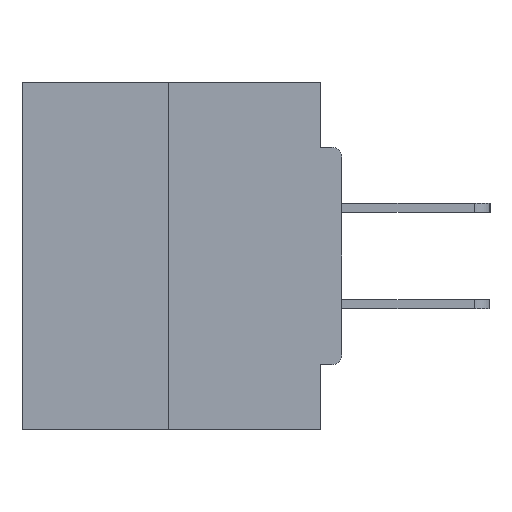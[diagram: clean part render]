
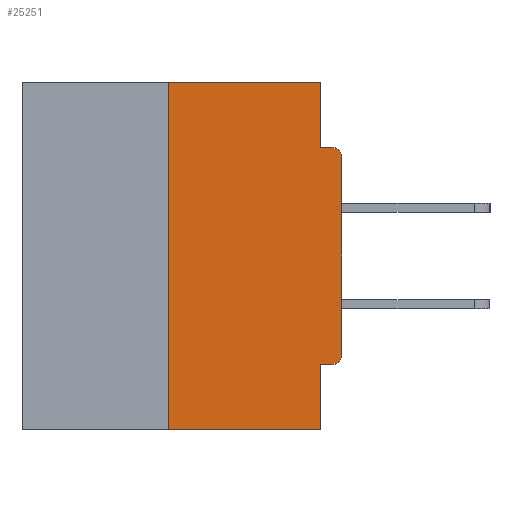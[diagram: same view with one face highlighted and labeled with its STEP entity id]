
A CAD part, left-side view. The second image highlights one B-rep face of the part: STEP entity #25251.
In plain terms, the highlighted planar face has unit normal (-1, 0, 0).
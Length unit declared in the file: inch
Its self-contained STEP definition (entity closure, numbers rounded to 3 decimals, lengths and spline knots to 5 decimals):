
#108 = ORIENTED_EDGE ( 'NONE', *, *, #28873, .F. ) ;
#374 = VERTEX_POINT ( 'NONE', #25439 ) ;
#967 = VECTOR ( 'NONE', #21039, 39.37008 ) ;
#1845 = VERTEX_POINT ( 'NONE', #27492 ) ;
#2321 = LINE ( 'NONE', #20231, #15808 ) ;
#3077 = AXIS2_PLACEMENT_3D ( 'NONE', #6967, #7085, #28451 ) ;
#3712 = CARTESIAN_POINT ( 'NONE',  ( 0., 0.015, -0.4065 ) ) ;
#3963 = VERTEX_POINT ( 'NONE', #11438 ) ;
#4466 = CARTESIAN_POINT ( 'NONE',  ( 0., 0.25, 0. ) ) ;
#4668 = VECTOR ( 'NONE', #16037, 39.37008 ) ;
#4736 = LINE ( 'NONE', #13204, #967 ) ;
#4924 = EDGE_CURVE ( 'NONE', #24156, #24502, #10469, .T. ) ;
#5643 = DIRECTION ( 'NONE',  ( 0., 0., -1. ) ) ;
#5819 = DIRECTION ( 'NONE',  ( -1., 0., 0. ) ) ;
#5841 = VECTOR ( 'NONE', #5643, 39.37008 ) ;
#5943 = DIRECTION ( 'NONE',  ( 0., 0., 1. ) ) ;
#6967 = CARTESIAN_POINT ( 'NONE',  ( 0., 0.015, -0.1085 ) ) ;
#7085 = DIRECTION ( 'NONE',  ( -1., 0., 0. ) ) ;
#8122 = VERTEX_POINT ( 'NONE', #13947 ) ;
#8282 = ORIENTED_EDGE ( 'NONE', *, *, #14722, .T. ) ;
#8431 = LINE ( 'NONE', #8628, #26182 ) ;
#8519 = EDGE_CURVE ( 'NONE', #18077, #1845, #4736, .T. ) ;
#8626 = CARTESIAN_POINT ( 'NONE',  ( 0., 0.031, -0.5 ) ) ;
#8628 = CARTESIAN_POINT ( 'NONE',  ( 0., 0., -0.0935 ) ) ;
#9021 = ORIENTED_EDGE ( 'NONE', *, *, #8519, .F. ) ;
#9409 = ORIENTED_EDGE ( 'NONE', *, *, #18196, .T. ) ;
#9428 = EDGE_CURVE ( 'NONE', #374, #25283, #22855, .T. ) ;
#10469 = LINE ( 'NONE', #32839, #5841 ) ;
#10482 = ORIENTED_EDGE ( 'NONE', *, *, #20286, .F. ) ;
#10973 = CARTESIAN_POINT ( 'NONE',  ( 0., 0.25, 0. ) ) ;
#11276 = CARTESIAN_POINT ( 'NONE',  ( 0., 0., -0.3915 ) ) ;
#11438 = CARTESIAN_POINT ( 'NONE',  ( 0., 0.015, -0.0935 ) ) ;
#12841 = DIRECTION ( 'NONE',  ( 0., 0., -1. ) ) ;
#13204 = CARTESIAN_POINT ( 'NONE',  ( 0., 0.031, 0. ) ) ;
#13947 = CARTESIAN_POINT ( 'NONE',  ( 0., 0., -0.1085 ) ) ;
#14625 = DIRECTION ( 'NONE',  ( 0., -1., 0. ) ) ;
#14722 = EDGE_CURVE ( 'NONE', #8122, #3963, #25601, .T. ) ;
#15189 = DIRECTION ( 'NONE',  ( 1., 0., 0. ) ) ;
#15808 = VECTOR ( 'NONE', #17378, 39.37008 ) ;
#16037 = DIRECTION ( 'NONE',  ( 0., 0., 1. ) ) ;
#17378 = DIRECTION ( 'NONE',  ( 0., 1., 0. ) ) ;
#17781 = LINE ( 'NONE', #19398, #21137 ) ;
#18077 = VERTEX_POINT ( 'NONE', #18548 ) ;
#18196 = EDGE_CURVE ( 'NONE', #19722, #8122, #17781, .T. ) ;
#18548 = CARTESIAN_POINT ( 'NONE',  ( 0., 0.031, 0. ) ) ;
#18987 = EDGE_CURVE ( 'NONE', #1845, #3963, #8431, .T. ) ;
#19374 = EDGE_CURVE ( 'NONE', #28851, #19722, #34179, .T. ) ;
#19398 = CARTESIAN_POINT ( 'NONE',  ( 0., 0., 0. ) ) ;
#19722 = VERTEX_POINT ( 'NONE', #11276 ) ;
#20144 = VECTOR ( 'NONE', #14625, 39.37008 ) ;
#20173 = VECTOR ( 'NONE', #32762, 39.37008 ) ;
#20231 = CARTESIAN_POINT ( 'NONE',  ( 0., 0., -0.4065 ) ) ;
#20286 = EDGE_CURVE ( 'NONE', #25283, #18077, #28169, .T. ) ;
#20977 = AXIS2_PLACEMENT_3D ( 'NONE', #29039, #15189, #12841 ) ;
#21012 = LINE ( 'NONE', #22252, #20173 ) ;
#21039 = DIRECTION ( 'NONE',  ( 0., 0., -1. ) ) ;
#21137 = VECTOR ( 'NONE', #5943, 39.37008 ) ;
#21231 = EDGE_LOOP ( 'NONE', ( #10482, #34613, #34446, #22995, #108, #27698, #9409, #8282, #28003, #9021 ) ) ;
#21971 = DIRECTION ( 'NONE',  ( 0., -1., 0. ) ) ;
#22252 = CARTESIAN_POINT ( 'NONE',  ( 0., 0.46, -0.5 ) ) ;
#22855 = LINE ( 'NONE', #10973, #4668 ) ;
#22995 = ORIENTED_EDGE ( 'NONE', *, *, #4924, .F. ) ;
#24156 = VERTEX_POINT ( 'NONE', #26345 ) ;
#24502 = VERTEX_POINT ( 'NONE', #8626 ) ;
#25251 = ADVANCED_FACE ( 'NONE', ( #32556 ), #31409, .F. ) ;
#25283 = VERTEX_POINT ( 'NONE', #4466 ) ;
#25439 = CARTESIAN_POINT ( 'NONE',  ( 0., 0.25, -0.5 ) ) ;
#25601 = CIRCLE ( 'NONE', #3077, 0.015 ) ;
#26182 = VECTOR ( 'NONE', #21971, 39.37008 ) ;
#26345 = CARTESIAN_POINT ( 'NONE',  ( 0., 0.031, -0.4065 ) ) ;
#26979 = EDGE_CURVE ( 'NONE', #374, #24502, #21012, .T. ) ;
#27492 = CARTESIAN_POINT ( 'NONE',  ( 0., 0.031, -0.0935 ) ) ;
#27698 = ORIENTED_EDGE ( 'NONE', *, *, #19374, .T. ) ;
#28003 = ORIENTED_EDGE ( 'NONE', *, *, #18987, .F. ) ;
#28169 = LINE ( 'NONE', #30706, #20144 ) ;
#28451 = DIRECTION ( 'NONE',  ( 0., 0., -1. ) ) ;
#28851 = VERTEX_POINT ( 'NONE', #3712 ) ;
#28873 = EDGE_CURVE ( 'NONE', #28851, #24156, #2321, .T. ) ;
#29039 = CARTESIAN_POINT ( 'NONE',  ( 0., 0.46, 0. ) ) ;
#29903 = DIRECTION ( 'NONE',  ( 0., 0., -1. ) ) ;
#30706 = CARTESIAN_POINT ( 'NONE',  ( 0., 0.46, 0. ) ) ;
#31409 = PLANE ( 'NONE',  #20977 ) ;
#31969 = AXIS2_PLACEMENT_3D ( 'NONE', #32642, #5819, #29903 ) ;
#32556 = FACE_OUTER_BOUND ( 'NONE', #21231, .T. ) ;
#32642 = CARTESIAN_POINT ( 'NONE',  ( 0., 0.015, -0.3915 ) ) ;
#32762 = DIRECTION ( 'NONE',  ( 0., -1., 0. ) ) ;
#32839 = CARTESIAN_POINT ( 'NONE',  ( 0., 0.031, -0.5 ) ) ;
#34179 = CIRCLE ( 'NONE', #31969, 0.015 ) ;
#34446 = ORIENTED_EDGE ( 'NONE', *, *, #26979, .T. ) ;
#34613 = ORIENTED_EDGE ( 'NONE', *, *, #9428, .F. ) ;
